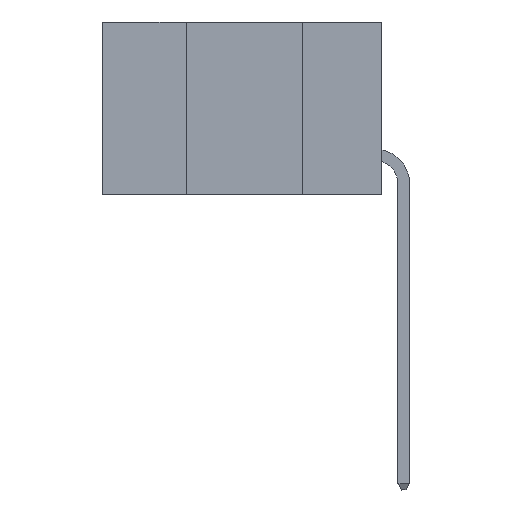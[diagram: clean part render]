
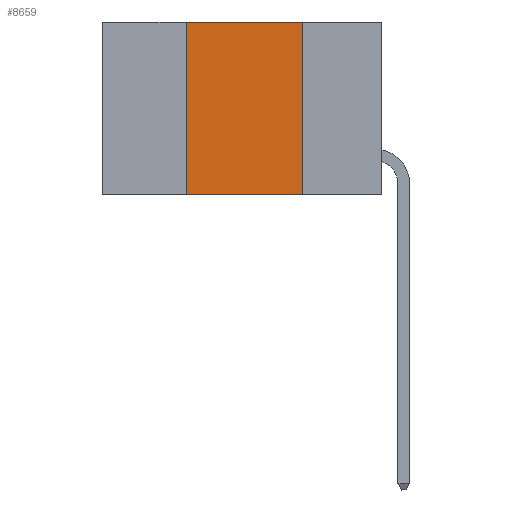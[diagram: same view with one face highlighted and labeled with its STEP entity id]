
A CAD part, left-side view. The second image highlights one B-rep face of the part: STEP entity #8659.
In plain terms, the highlighted planar face has unit normal (-1, 0, 0).
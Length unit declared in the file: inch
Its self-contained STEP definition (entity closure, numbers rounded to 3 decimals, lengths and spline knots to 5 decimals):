
#150 = CARTESIAN_POINT ( 'NONE',  ( 0., 0.6, -0.37 ) ) ;
#574 = DIRECTION ( 'NONE',  ( 0., -1., 0. ) ) ;
#712 = CARTESIAN_POINT ( 'NONE',  ( 0., 0.17, -0.37 ) ) ;
#1278 = DIRECTION ( 'NONE',  ( 0., 0., -1. ) ) ;
#1556 = CARTESIAN_POINT ( 'NONE',  ( 0., 0.6, 0. ) ) ;
#1648 = DIRECTION ( 'NONE',  ( 1., 0., 0. ) ) ;
#1824 = VERTEX_POINT ( 'NONE', #7685 ) ;
#2122 = LINE ( 'NONE', #6514, #6227 ) ;
#2641 = EDGE_CURVE ( 'NONE', #4918, #6188, #6639, .T. ) ;
#3884 = ORIENTED_EDGE ( 'NONE', *, *, #22384, .F. ) ;
#4918 = VERTEX_POINT ( 'NONE', #19111 ) ;
#5820 = LINE ( 'NONE', #8378, #15310 ) ;
#6188 = VERTEX_POINT ( 'NONE', #712 ) ;
#6227 = VECTOR ( 'NONE', #574, 39.37008 ) ;
#6514 = CARTESIAN_POINT ( 'NONE',  ( 0., 0.6, 0. ) ) ;
#6639 = LINE ( 'NONE', #150, #23160 ) ;
#6709 = DIRECTION ( 'NONE',  ( 0., -1., 0. ) ) ;
#7685 = CARTESIAN_POINT ( 'NONE',  ( 0., 0.42, 0. ) ) ;
#8378 = CARTESIAN_POINT ( 'NONE',  ( 0., 0.42, 0. ) ) ;
#8659 = ADVANCED_FACE ( 'NONE', ( #20067 ), #9701, .F. ) ;
#9691 = CARTESIAN_POINT ( 'NONE',  ( 0., 0.17, 0. ) ) ;
#9701 = PLANE ( 'NONE',  #22382 ) ;
#9732 = VECTOR ( 'NONE', #14433, 39.37008 ) ;
#11262 = ORIENTED_EDGE ( 'NONE', *, *, #18824, .F. ) ;
#12353 = CARTESIAN_POINT ( 'NONE',  ( 0., 0.17, 0. ) ) ;
#13040 = ORIENTED_EDGE ( 'NONE', *, *, #24907, .F. ) ;
#14433 = DIRECTION ( 'NONE',  ( 0., 0., -1. ) ) ;
#14480 = EDGE_LOOP ( 'NONE', ( #3884, #11262, #13040, #20924 ) ) ;
#15310 = VECTOR ( 'NONE', #24886, 39.37008 ) ;
#18824 = EDGE_CURVE ( 'NONE', #1824, #22814, #2122, .T. ) ;
#19111 = CARTESIAN_POINT ( 'NONE',  ( 0., 0.42, -0.37 ) ) ;
#19935 = LINE ( 'NONE', #12353, #9732 ) ;
#20067 = FACE_OUTER_BOUND ( 'NONE', #14480, .T. ) ;
#20924 = ORIENTED_EDGE ( 'NONE', *, *, #2641, .T. ) ;
#22382 = AXIS2_PLACEMENT_3D ( 'NONE', #1556, #1648, #1278 ) ;
#22384 = EDGE_CURVE ( 'NONE', #22814, #6188, #19935, .T. ) ;
#22814 = VERTEX_POINT ( 'NONE', #9691 ) ;
#23160 = VECTOR ( 'NONE', #6709, 39.37008 ) ;
#24886 = DIRECTION ( 'NONE',  ( 0., 0., 1. ) ) ;
#24907 = EDGE_CURVE ( 'NONE', #4918, #1824, #5820, .T. ) ;
